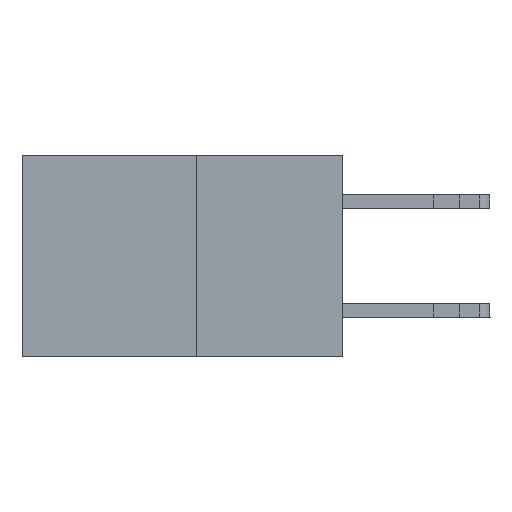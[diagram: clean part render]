
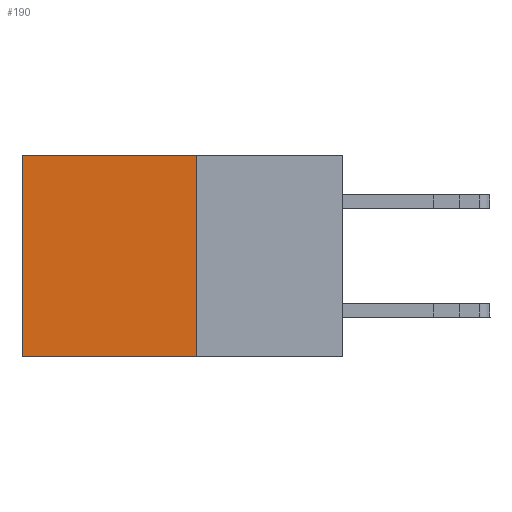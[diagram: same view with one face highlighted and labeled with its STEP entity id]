
A CAD part, left-side view. The second image highlights one B-rep face of the part: STEP entity #190.
In plain terms, the highlighted planar face has unit normal (-1, 0, 0).
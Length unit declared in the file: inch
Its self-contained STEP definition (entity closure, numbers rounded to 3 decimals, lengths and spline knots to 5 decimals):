
#190 = ADVANCED_FACE ( 'NONE', ( #1288 ), #3224, .F. ) ;
#1288 = FACE_OUTER_BOUND ( 'NONE', #22356, .T. ) ;
#1443 = LINE ( 'NONE', #10672, #15899 ) ;
#1483 = ORIENTED_EDGE ( 'NONE', *, *, #23862, .T. ) ;
#1509 = EDGE_CURVE ( 'NONE', #18449, #21256, #7699, .T. ) ;
#1689 = DIRECTION ( 'NONE',  ( 0., 0., -1. ) ) ;
#1911 = CARTESIAN_POINT ( 'NONE',  ( 0.277, 0.59, 0. ) ) ;
#2908 = LINE ( 'NONE', #8772, #17980 ) ;
#2934 = ORIENTED_EDGE ( 'NONE', *, *, #14668, .F. ) ;
#3224 = PLANE ( 'NONE',  #4220 ) ;
#3888 = CARTESIAN_POINT ( 'NONE',  ( 0.277, 0.27, -0.37 ) ) ;
#4220 = AXIS2_PLACEMENT_3D ( 'NONE', #3888, #8297, #1689 ) ;
#5246 = LINE ( 'NONE', #19891, #10207 ) ;
#7699 = LINE ( 'NONE', #11563, #17144 ) ;
#8297 = DIRECTION ( 'NONE',  ( 1., 0., 0. ) ) ;
#8752 = VERTEX_POINT ( 'NONE', #1911 ) ;
#8772 = CARTESIAN_POINT ( 'NONE',  ( 0.277, 0.27, -0.37 ) ) ;
#9679 = VERTEX_POINT ( 'NONE', #17888 ) ;
#10207 = VECTOR ( 'NONE', #16066, 39.37008 ) ;
#10672 = CARTESIAN_POINT ( 'NONE',  ( 0.277, 0.27, 0. ) ) ;
#10684 = DIRECTION ( 'NONE',  ( 0., 0., -1. ) ) ;
#10792 = CARTESIAN_POINT ( 'NONE',  ( 0.277, 0.59, -0.37 ) ) ;
#10890 = EDGE_CURVE ( 'NONE', #8752, #21256, #5246, .T. ) ;
#11405 = DIRECTION ( 'NONE',  ( 0., 1., 0. ) ) ;
#11563 = CARTESIAN_POINT ( 'NONE',  ( 0.277, 0.27, -0.37 ) ) ;
#14668 = EDGE_CURVE ( 'NONE', #9679, #18449, #2908, .T. ) ;
#14882 = ORIENTED_EDGE ( 'NONE', *, *, #1509, .F. ) ;
#14930 = ORIENTED_EDGE ( 'NONE', *, *, #10890, .T. ) ;
#15899 = VECTOR ( 'NONE', #20187, 39.37008 ) ;
#16066 = DIRECTION ( 'NONE',  ( 0., 0., -1. ) ) ;
#17072 = CARTESIAN_POINT ( 'NONE',  ( 0.277, 0.27, -0.37 ) ) ;
#17144 = VECTOR ( 'NONE', #11405, 39.37008 ) ;
#17888 = CARTESIAN_POINT ( 'NONE',  ( 0.277, 0.27, 0. ) ) ;
#17980 = VECTOR ( 'NONE', #10684, 39.37008 ) ;
#18449 = VERTEX_POINT ( 'NONE', #17072 ) ;
#19891 = CARTESIAN_POINT ( 'NONE',  ( 0.277, 0.59, -0.37 ) ) ;
#20187 = DIRECTION ( 'NONE',  ( 0., 1., 0. ) ) ;
#21256 = VERTEX_POINT ( 'NONE', #10792 ) ;
#22356 = EDGE_LOOP ( 'NONE', ( #14930, #14882, #2934, #1483 ) ) ;
#23862 = EDGE_CURVE ( 'NONE', #9679, #8752, #1443, .T. ) ;
